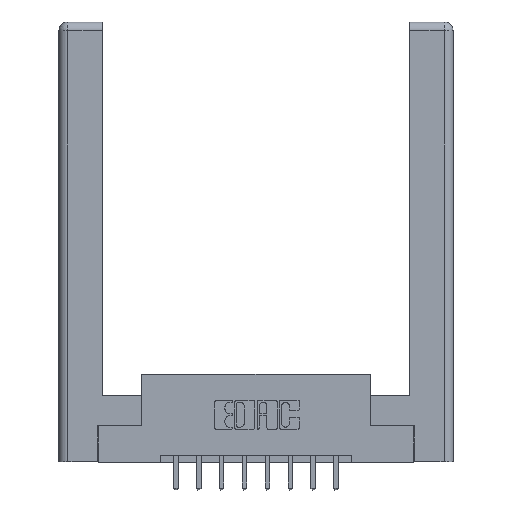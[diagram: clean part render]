
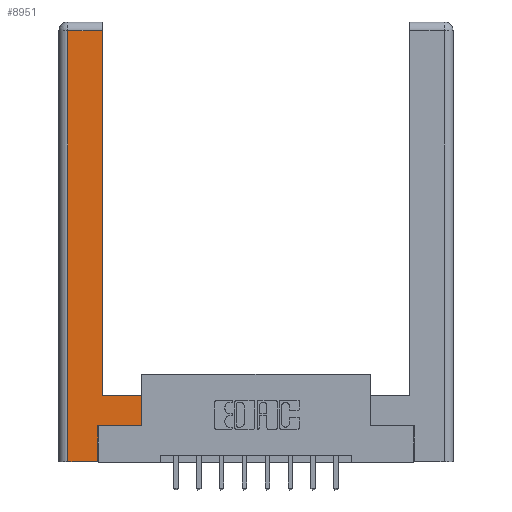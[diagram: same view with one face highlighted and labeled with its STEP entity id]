
A CAD part, top view. The second image highlights one B-rep face of the part: STEP entity #8951.
In plain terms, the highlighted planar face has unit normal (0, 0, 1).
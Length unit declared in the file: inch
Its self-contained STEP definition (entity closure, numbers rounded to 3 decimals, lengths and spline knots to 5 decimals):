
#219 = CARTESIAN_POINT ( 'NONE',  ( 0.565, 0.245, 0. ) ) ;
#345 = LINE ( 'NONE', #2523, #1787 ) ;
#1103 = ORIENTED_EDGE ( 'NONE', *, *, #8893, .T. ) ;
#1482 = LINE ( 'NONE', #9257, #6663 ) ;
#1625 = CARTESIAN_POINT ( 'NONE',  ( 0.295, 0.45, 0. ) ) ;
#1787 = VECTOR ( 'NONE', #12649, 39.37008 ) ;
#2141 = VERTEX_POINT ( 'NONE', #10326 ) ;
#2288 = VERTEX_POINT ( 'NONE', #219 ) ;
#2297 = CARTESIAN_POINT ( 'NONE',  ( 0.295, 0.45, 0. ) ) ;
#2523 = CARTESIAN_POINT ( 'NONE',  ( 0.565, 0.45, 0. ) ) ;
#2670 = VECTOR ( 'NONE', #12025, 39.37008 ) ;
#2841 = PLANE ( 'NONE',  #12457 ) ;
#2842 = VECTOR ( 'NONE', #3770, 39.37008 ) ;
#2852 = CARTESIAN_POINT ( 'NONE',  ( 0.0615, 0., 0. ) ) ;
#2914 = CARTESIAN_POINT ( 'NONE',  ( 0.565, 0.45, 0. ) ) ;
#3012 = EDGE_CURVE ( 'NONE', #3683, #2141, #12285, .T. ) ;
#3683 = VERTEX_POINT ( 'NONE', #8615 ) ;
#3691 = EDGE_CURVE ( 'NONE', #5113, #5301, #5323, .T. ) ;
#3770 = DIRECTION ( 'NONE',  ( -1., 0., 0. ) ) ;
#3948 = VERTEX_POINT ( 'NONE', #2914 ) ;
#3960 = DIRECTION ( 'NONE',  ( 1., 0., 0. ) ) ;
#4134 = CARTESIAN_POINT ( 'NONE',  ( 0.295, 3., 0. ) ) ;
#4347 = VECTOR ( 'NONE', #6001, 39.37008 ) ;
#4613 = VECTOR ( 'NONE', #11576, 39.37008 ) ;
#4936 = VERTEX_POINT ( 'NONE', #2297 ) ;
#4951 = CARTESIAN_POINT ( 'NONE',  ( 0.265, 0.245, 0. ) ) ;
#5113 = VERTEX_POINT ( 'NONE', #5190 ) ;
#5190 = CARTESIAN_POINT ( 'NONE',  ( 0.295, 2.94, 0. ) ) ;
#5301 = VERTEX_POINT ( 'NONE', #9365 ) ;
#5323 = LINE ( 'NONE', #9636, #6774 ) ;
#6001 = DIRECTION ( 'NONE',  ( 0., 1., 0. ) ) ;
#6214 = EDGE_CURVE ( 'NONE', #3948, #4936, #7710, .T. ) ;
#6663 = VECTOR ( 'NONE', #8220, 39.37008 ) ;
#6774 = VECTOR ( 'NONE', #10739, 39.37008 ) ;
#7232 = LINE ( 'NONE', #7970, #2670 ) ;
#7710 = LINE ( 'NONE', #1625, #2842 ) ;
#7970 = CARTESIAN_POINT ( 'NONE',  ( 0.565, 0.245, 0. ) ) ;
#8220 = DIRECTION ( 'NONE',  ( 0., -1., 0. ) ) ;
#8520 = EDGE_CURVE ( 'NONE', #5301, #11621, #1482, .T. ) ;
#8615 = CARTESIAN_POINT ( 'NONE',  ( 0.265, 0., 0. ) ) ;
#8893 = EDGE_CURVE ( 'NONE', #2288, #3948, #345, .T. ) ;
#8951 = ADVANCED_FACE ( 'NONE', ( #13111 ), #2841, .F. ) ;
#9019 = ORIENTED_EDGE ( 'NONE', *, *, #13287, .T. ) ;
#9099 = ORIENTED_EDGE ( 'NONE', *, *, #6214, .T. ) ;
#9148 = CARTESIAN_POINT ( 'NONE',  ( 0., 0., 0. ) ) ;
#9155 = LINE ( 'NONE', #4134, #4613 ) ;
#9190 = DIRECTION ( 'NONE',  ( -1., 0., 0. ) ) ;
#9257 = CARTESIAN_POINT ( 'NONE',  ( 0.0615, 0., 0. ) ) ;
#9365 = CARTESIAN_POINT ( 'NONE',  ( 0.0615, 2.94, 0. ) ) ;
#9636 = CARTESIAN_POINT ( 'NONE',  ( 0.0615, 2.94, 0. ) ) ;
#9642 = ORIENTED_EDGE ( 'NONE', *, *, #12770, .T. ) ;
#10133 = ORIENTED_EDGE ( 'NONE', *, *, #3012, .T. ) ;
#10326 = CARTESIAN_POINT ( 'NONE',  ( 0.265, 0.245, 0. ) ) ;
#10705 = ORIENTED_EDGE ( 'NONE', *, *, #3691, .T. ) ;
#10739 = DIRECTION ( 'NONE',  ( -1., 0., 0. ) ) ;
#10959 = EDGE_LOOP ( 'NONE', ( #9019, #10705, #11395, #13167, #10133, #9642, #1103, #9099 ) ) ;
#11355 = CARTESIAN_POINT ( 'NONE',  ( 0.265, 0., 0. ) ) ;
#11395 = ORIENTED_EDGE ( 'NONE', *, *, #8520, .T. ) ;
#11576 = DIRECTION ( 'NONE',  ( 0., 1., 0. ) ) ;
#11621 = VERTEX_POINT ( 'NONE', #2852 ) ;
#11902 = VECTOR ( 'NONE', #3960, 39.37008 ) ;
#12025 = DIRECTION ( 'NONE',  ( 1., 0., 0. ) ) ;
#12245 = DIRECTION ( 'NONE',  ( 0., 0., -1. ) ) ;
#12285 = LINE ( 'NONE', #4951, #4347 ) ;
#12376 = LINE ( 'NONE', #11355, #11902 ) ;
#12457 = AXIS2_PLACEMENT_3D ( 'NONE', #9148, #12245, #9190 ) ;
#12649 = DIRECTION ( 'NONE',  ( 0., 1., 0. ) ) ;
#12770 = EDGE_CURVE ( 'NONE', #2141, #2288, #7232, .T. ) ;
#12856 = EDGE_CURVE ( 'NONE', #11621, #3683, #12376, .T. ) ;
#13111 = FACE_OUTER_BOUND ( 'NONE', #10959, .T. ) ;
#13167 = ORIENTED_EDGE ( 'NONE', *, *, #12856, .T. ) ;
#13287 = EDGE_CURVE ( 'NONE', #4936, #5113, #9155, .T. ) ;
